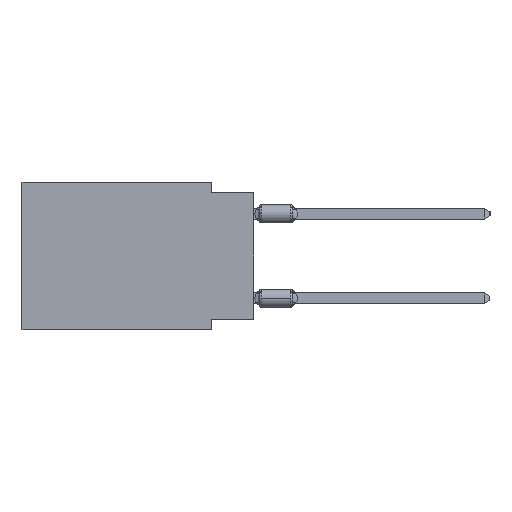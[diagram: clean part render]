
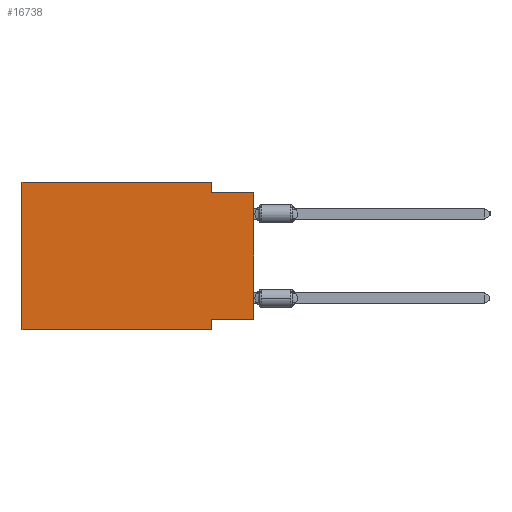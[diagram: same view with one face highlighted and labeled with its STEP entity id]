
A CAD part, left-side view. The second image highlights one B-rep face of the part: STEP entity #16738.
In plain terms, the highlighted planar face has unit normal (-1, 0, 0).
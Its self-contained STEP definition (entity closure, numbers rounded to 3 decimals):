
#1352 = EDGE_CURVE ( 'NONE', #23961, #18017, #14908, .T. ) ;
#1462 = CARTESIAN_POINT ( 'NONE',  ( 0., 13.97, 0. ) ) ;
#2041 = DIRECTION ( 'NONE',  ( 0., 0., -1. ) ) ;
#2192 = VERTEX_POINT ( 'NONE', #12920 ) ;
#2664 = ORIENTED_EDGE ( 'NONE', *, *, #2775, .F. ) ;
#2775 = EDGE_CURVE ( 'NONE', #2192, #6081, #30961, .T. ) ;
#3613 = PLANE ( 'NONE',  #9813 ) ;
#3965 = CARTESIAN_POINT ( 'NONE',  ( 0., 2.54, -8.89 ) ) ;
#4397 = ORIENTED_EDGE ( 'NONE', *, *, #16153, .T. ) ;
#4534 = LINE ( 'NONE', #17479, #14326 ) ;
#5069 = CARTESIAN_POINT ( 'NONE',  ( 0., 0., -8.255 ) ) ;
#5277 = CARTESIAN_POINT ( 'NONE',  ( 0., 2.54, -8.89 ) ) ;
#5563 = CARTESIAN_POINT ( 'NONE',  ( 0., 0., -0.635 ) ) ;
#5748 = CARTESIAN_POINT ( 'NONE',  ( 0., 13.97, -8.89 ) ) ;
#6081 = VERTEX_POINT ( 'NONE', #28393 ) ;
#6628 = VERTEX_POINT ( 'NONE', #5563 ) ;
#7268 = CARTESIAN_POINT ( 'NONE',  ( 0., 0., 0. ) ) ;
#7645 = CARTESIAN_POINT ( 'NONE',  ( 0., 0., -8.255 ) ) ;
#8398 = VECTOR ( 'NONE', #20755, 1000. ) ;
#8500 = EDGE_CURVE ( 'NONE', #34007, #2192, #4534, .T. ) ;
#8715 = ORIENTED_EDGE ( 'NONE', *, *, #8500, .F. ) ;
#8947 = CARTESIAN_POINT ( 'NONE',  ( 0., 2.54, 0. ) ) ;
#9219 = VECTOR ( 'NONE', #9448, 1000. ) ;
#9253 = ORIENTED_EDGE ( 'NONE', *, *, #10283, .F. ) ;
#9448 = DIRECTION ( 'NONE',  ( 0., 0., -1. ) ) ;
#9667 = ORIENTED_EDGE ( 'NONE', *, *, #27708, .T. ) ;
#9813 = AXIS2_PLACEMENT_3D ( 'NONE', #23422, #15319, #20316 ) ;
#10283 = EDGE_CURVE ( 'NONE', #6081, #15911, #22047, .T. ) ;
#12920 = CARTESIAN_POINT ( 'NONE',  ( 0., 13.97, 0. ) ) ;
#14326 = VECTOR ( 'NONE', #25593, 1000. ) ;
#14589 = CARTESIAN_POINT ( 'NONE',  ( 0., 2.54, -8.255 ) ) ;
#14656 = CARTESIAN_POINT ( 'NONE',  ( 0., 13.97, -8.89 ) ) ;
#14908 = LINE ( 'NONE', #5069, #15504 ) ;
#15319 = DIRECTION ( 'NONE',  ( 1., 0., 0. ) ) ;
#15504 = VECTOR ( 'NONE', #28030, 1000. ) ;
#15911 = VERTEX_POINT ( 'NONE', #25132 ) ;
#16153 = EDGE_CURVE ( 'NONE', #34007, #23587, #21600, .T. ) ;
#16435 = DIRECTION ( 'NONE',  ( 0., -1., 0. ) ) ;
#16586 = ORIENTED_EDGE ( 'NONE', *, *, #1352, .F. ) ;
#16738 = ADVANCED_FACE ( 'NONE', ( #27274 ), #3613, .F. ) ;
#17455 = DIRECTION ( 'NONE',  ( 0., 0., 1. ) ) ;
#17479 = CARTESIAN_POINT ( 'NONE',  ( 0., 13.97, 0. ) ) ;
#18017 = VERTEX_POINT ( 'NONE', #14589 ) ;
#18780 = ORIENTED_EDGE ( 'NONE', *, *, #33335, .F. ) ;
#18997 = VECTOR ( 'NONE', #17455, 1000. ) ;
#20316 = DIRECTION ( 'NONE',  ( 0., 0., -1. ) ) ;
#20755 = DIRECTION ( 'NONE',  ( 0., -1., 0. ) ) ;
#21600 = LINE ( 'NONE', #5748, #31280 ) ;
#22047 = LINE ( 'NONE', #8947, #9219 ) ;
#23422 = CARTESIAN_POINT ( 'NONE',  ( 0., 13.97, 0. ) ) ;
#23587 = VERTEX_POINT ( 'NONE', #5277 ) ;
#23689 = CARTESIAN_POINT ( 'NONE',  ( 0., 0., -0.635 ) ) ;
#23961 = VERTEX_POINT ( 'NONE', #7645 ) ;
#24142 = ORIENTED_EDGE ( 'NONE', *, *, #24631, .F. ) ;
#24420 = VECTOR ( 'NONE', #30625, 1000. ) ;
#24631 = EDGE_CURVE ( 'NONE', #18017, #23587, #25527, .T. ) ;
#25132 = CARTESIAN_POINT ( 'NONE',  ( 0., 2.54, -0.635 ) ) ;
#25527 = LINE ( 'NONE', #3965, #33264 ) ;
#25593 = DIRECTION ( 'NONE',  ( 0., 0., 1. ) ) ;
#27274 = FACE_OUTER_BOUND ( 'NONE', #29430, .T. ) ;
#27708 = EDGE_CURVE ( 'NONE', #23961, #6628, #33497, .T. ) ;
#28030 = DIRECTION ( 'NONE',  ( 0., 1., 0. ) ) ;
#28393 = CARTESIAN_POINT ( 'NONE',  ( 0., 2.54, 0. ) ) ;
#29430 = EDGE_LOOP ( 'NONE', ( #9667, #18780, #9253, #2664, #8715, #4397, #24142, #16586 ) ) ;
#30625 = DIRECTION ( 'NONE',  ( 0., -1., 0. ) ) ;
#30961 = LINE ( 'NONE', #1462, #24420 ) ;
#31280 = VECTOR ( 'NONE', #16435, 1000. ) ;
#31975 = LINE ( 'NONE', #23689, #8398 ) ;
#33264 = VECTOR ( 'NONE', #2041, 1000. ) ;
#33335 = EDGE_CURVE ( 'NONE', #15911, #6628, #31975, .T. ) ;
#33497 = LINE ( 'NONE', #7268, #18997 ) ;
#34007 = VERTEX_POINT ( 'NONE', #14656 ) ;
